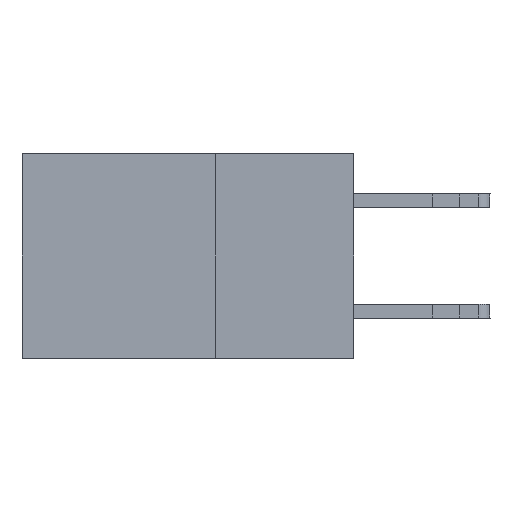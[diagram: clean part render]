
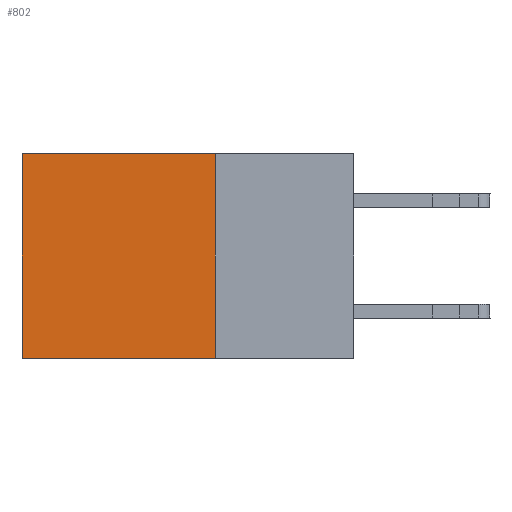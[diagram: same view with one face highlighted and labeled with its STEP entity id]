
A CAD part, left-side view. The second image highlights one B-rep face of the part: STEP entity #802.
In plain terms, the highlighted planar face has unit normal (-1, 0, 0).
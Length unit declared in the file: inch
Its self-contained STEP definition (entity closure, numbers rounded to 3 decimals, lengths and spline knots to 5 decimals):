
#219 = VERTEX_POINT ( 'NONE', #13230 ) ;
#802 = ADVANCED_FACE ( 'NONE', ( #3358 ), #9915, .F. ) ;
#1597 = DIRECTION ( 'NONE',  ( 0., 0., -1. ) ) ;
#1702 = LINE ( 'NONE', #20204, #9921 ) ;
#2379 = VERTEX_POINT ( 'NONE', #13079 ) ;
#2765 = EDGE_CURVE ( 'NONE', #219, #2379, #4098, .T. ) ;
#3358 = FACE_OUTER_BOUND ( 'NONE', #12702, .T. ) ;
#3397 = ORIENTED_EDGE ( 'NONE', *, *, #2765, .F. ) ;
#3540 = VECTOR ( 'NONE', #19513, 39.37008 ) ;
#3784 = AXIS2_PLACEMENT_3D ( 'NONE', #11665, #13537, #1597 ) ;
#4098 = LINE ( 'NONE', #19412, #3540 ) ;
#6743 = DIRECTION ( 'NONE',  ( 0., 1., 0. ) ) ;
#7716 = CARTESIAN_POINT ( 'NONE',  ( 0.2875, 0.6, 0. ) ) ;
#9877 = ORIENTED_EDGE ( 'NONE', *, *, #21068, .T. ) ;
#9915 = PLANE ( 'NONE',  #3784 ) ;
#9921 = VECTOR ( 'NONE', #6743, 39.37008 ) ;
#11201 = VECTOR ( 'NONE', #15150, 39.37008 ) ;
#11665 = CARTESIAN_POINT ( 'NONE',  ( 0.2875, 0.25, 0. ) ) ;
#11813 = ORIENTED_EDGE ( 'NONE', *, *, #17226, .T. ) ;
#11891 = CARTESIAN_POINT ( 'NONE',  ( 0.2875, 0.25, 0. ) ) ;
#12702 = EDGE_LOOP ( 'NONE', ( #11813, #3397, #16969, #9877 ) ) ;
#13079 = CARTESIAN_POINT ( 'NONE',  ( 0.2875, 0.6, -0.37 ) ) ;
#13230 = CARTESIAN_POINT ( 'NONE',  ( 0.2875, 0.25, -0.37 ) ) ;
#13537 = DIRECTION ( 'NONE',  ( 1., 0., 0. ) ) ;
#14203 = VERTEX_POINT ( 'NONE', #11891 ) ;
#14614 = CARTESIAN_POINT ( 'NONE',  ( 0.2875, 0.6, 0. ) ) ;
#15150 = DIRECTION ( 'NONE',  ( 0., 0., -1. ) ) ;
#15666 = EDGE_CURVE ( 'NONE', #14203, #219, #18653, .T. ) ;
#16189 = VECTOR ( 'NONE', #16372, 39.37008 ) ;
#16372 = DIRECTION ( 'NONE',  ( 0., 0., -1. ) ) ;
#16969 = ORIENTED_EDGE ( 'NONE', *, *, #15666, .F. ) ;
#17169 = VERTEX_POINT ( 'NONE', #7716 ) ;
#17226 = EDGE_CURVE ( 'NONE', #17169, #2379, #18333, .T. ) ;
#18333 = LINE ( 'NONE', #14614, #16189 ) ;
#18653 = LINE ( 'NONE', #20401, #11201 ) ;
#19412 = CARTESIAN_POINT ( 'NONE',  ( 0.2875, 0.25, -0.37 ) ) ;
#19513 = DIRECTION ( 'NONE',  ( 0., 1., 0. ) ) ;
#20204 = CARTESIAN_POINT ( 'NONE',  ( 0.2875, 0.25, 0. ) ) ;
#20401 = CARTESIAN_POINT ( 'NONE',  ( 0.2875, 0.25, 0. ) ) ;
#21068 = EDGE_CURVE ( 'NONE', #14203, #17169, #1702, .T. ) ;
